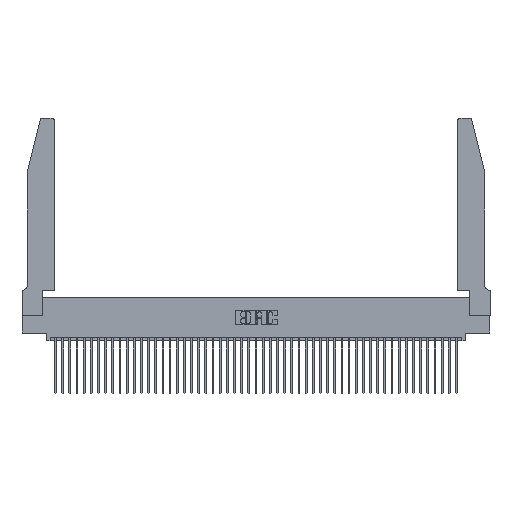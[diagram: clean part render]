
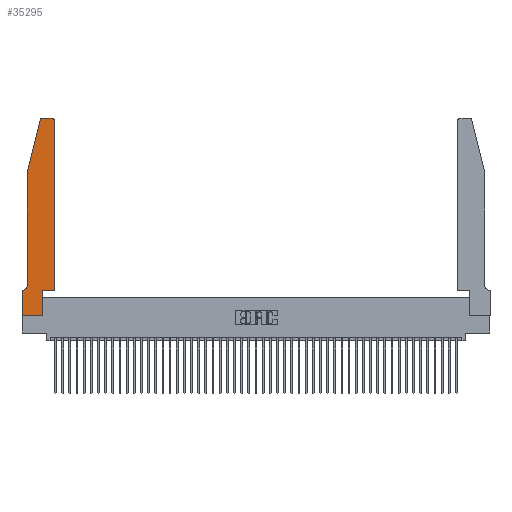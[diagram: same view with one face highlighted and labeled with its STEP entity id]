
A CAD part, top view. The second image highlights one B-rep face of the part: STEP entity #35295.
In plain terms, the highlighted planar face has unit normal (0, 0, 1).
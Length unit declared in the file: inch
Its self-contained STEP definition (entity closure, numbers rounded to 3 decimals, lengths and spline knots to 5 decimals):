
#497 = DIRECTION ( 'NONE',  ( -1., 0., 0. ) ) ;
#1406 = ORIENTED_EDGE ( 'NONE', *, *, #20816, .T. ) ;
#1784 = VECTOR ( 'NONE', #19630, 39.37008 ) ;
#1787 = VECTOR ( 'NONE', #44971, 39.37008 ) ;
#1931 = DIRECTION ( 'NONE',  ( -1., 0., 0. ) ) ;
#2581 = ORIENTED_EDGE ( 'NONE', *, *, #4898, .T. ) ;
#2944 = VERTEX_POINT ( 'NONE', #45969 ) ;
#3312 = CARTESIAN_POINT ( 'NONE',  ( 0., 0., 0.37 ) ) ;
#4297 = ORIENTED_EDGE ( 'NONE', *, *, #11537, .T. ) ;
#4477 = CARTESIAN_POINT ( 'NONE',  ( 0.2605, 2.75, 0.37 ) ) ;
#4898 = EDGE_CURVE ( 'NONE', #16310, #2944, #10769, .T. ) ;
#5303 = VECTOR ( 'NONE', #32879, 39.37008 ) ;
#5355 = CARTESIAN_POINT ( 'NONE',  ( 0.4505, 0.35, 0.37 ) ) ;
#5416 = VERTEX_POINT ( 'NONE', #45116 ) ;
#5475 = ORIENTED_EDGE ( 'NONE', *, *, #32530, .T. ) ;
#5559 = AXIS2_PLACEMENT_3D ( 'NONE', #45998, #24173, #1931 ) ;
#6091 = ORIENTED_EDGE ( 'NONE', *, *, #26059, .T. ) ;
#6346 = CARTESIAN_POINT ( 'NONE',  ( 0.284, 2.72, 0.37 ) ) ;
#6486 = VECTOR ( 'NONE', #18868, 39.37008 ) ;
#7063 = EDGE_LOOP ( 'NONE', ( #30308, #11888, #4297, #5475, #17757, #37172, #1406, #21222, #2581, #34363, #6091, #28052 ) ) ;
#7684 = VERTEX_POINT ( 'NONE', #38017 ) ;
#7776 = CIRCLE ( 'NONE', #23488, 0.03 ) ;
#8033 = EDGE_CURVE ( 'NONE', #5416, #16310, #46451, .T. ) ;
#9741 = LINE ( 'NONE', #5355, #36792 ) ;
#10107 = DIRECTION ( 'NONE',  ( 1., 0., 0. ) ) ;
#10769 = LINE ( 'NONE', #24474, #38880 ) ;
#10992 = CARTESIAN_POINT ( 'NONE',  ( 0.4505, 2.72, 0.37 ) ) ;
#11537 = EDGE_CURVE ( 'NONE', #7684, #43805, #45530, .T. ) ;
#11857 = VECTOR ( 'NONE', #497, 39.37008 ) ;
#11888 = ORIENTED_EDGE ( 'NONE', *, *, #41036, .T. ) ;
#12691 = VECTOR ( 'NONE', #44970, 39.37008 ) ;
#13039 = LINE ( 'NONE', #33638, #11857 ) ;
#13685 = CARTESIAN_POINT ( 'NONE',  ( 0., 0.35, 0.37 ) ) ;
#14522 = CARTESIAN_POINT ( 'NONE',  ( 0.0755, 0.42, 0.37 ) ) ;
#15375 = VERTEX_POINT ( 'NONE', #14522 ) ;
#15816 = CARTESIAN_POINT ( 'NONE',  ( 0.0055, 0.35, 0.37 ) ) ;
#15893 = CARTESIAN_POINT ( 'NONE',  ( 0.0755, 2., 0.37 ) ) ;
#16060 = CARTESIAN_POINT ( 'NONE',  ( 0.284, 2.75, 0.37 ) ) ;
#16310 = VERTEX_POINT ( 'NONE', #17488 ) ;
#16638 = EDGE_CURVE ( 'NONE', #19144, #25656, #13039, .T. ) ;
#17291 = CARTESIAN_POINT ( 'NONE',  ( 0., 0.35, 0.37 ) ) ;
#17488 = CARTESIAN_POINT ( 'NONE',  ( 0.2865, 0., 0.37 ) ) ;
#17757 = ORIENTED_EDGE ( 'NONE', *, *, #29373, .T. ) ;
#18868 = DIRECTION ( 'NONE',  ( -0.239, -0.971, 0. ) ) ;
#19128 = CIRCLE ( 'NONE', #46783, 0.03 ) ;
#19144 = VERTEX_POINT ( 'NONE', #15816 ) ;
#19630 = DIRECTION ( 'NONE',  ( 0., -1., 0. ) ) ;
#20816 = EDGE_CURVE ( 'NONE', #25656, #5416, #23893, .T. ) ;
#20916 = DIRECTION ( 'NONE',  ( 0., 0., 1. ) ) ;
#21017 = DIRECTION ( 'NONE',  ( 0., 0., 1. ) ) ;
#21222 = ORIENTED_EDGE ( 'NONE', *, *, #8033, .T. ) ;
#21611 = LINE ( 'NONE', #15893, #1784 ) ;
#22390 = VERTEX_POINT ( 'NONE', #16060 ) ;
#23488 = AXIS2_PLACEMENT_3D ( 'NONE', #42720, #20916, #46395 ) ;
#23893 = LINE ( 'NONE', #3312, #5303 ) ;
#24173 = DIRECTION ( 'NONE',  ( 0., 0., -1. ) ) ;
#24474 = CARTESIAN_POINT ( 'NONE',  ( 0.2865, 0.35, 0.37 ) ) ;
#25421 = DIRECTION ( 'NONE',  ( 1., 0., 0. ) ) ;
#25656 = VERTEX_POINT ( 'NONE', #13685 ) ;
#26059 = EDGE_CURVE ( 'NONE', #31080, #30648, #31266, .T. ) ;
#27065 = VECTOR ( 'NONE', #25421, 39.37008 ) ;
#28052 = ORIENTED_EDGE ( 'NONE', *, *, #36757, .T. ) ;
#28691 = VERTEX_POINT ( 'NONE', #37899 ) ;
#29373 = EDGE_CURVE ( 'NONE', #15375, #19144, #43479, .T. ) ;
#29726 = CARTESIAN_POINT ( 'NONE',  ( 0.0755, 2., 0.37 ) ) ;
#30308 = ORIENTED_EDGE ( 'NONE', *, *, #34353, .T. ) ;
#30330 = CARTESIAN_POINT ( 'NONE',  ( 0.4505, 0.35, 0.37 ) ) ;
#30648 = VERTEX_POINT ( 'NONE', #10992 ) ;
#31073 = LINE ( 'NONE', #4477, #12691 ) ;
#31080 = VERTEX_POINT ( 'NONE', #43634 ) ;
#31266 = LINE ( 'NONE', #30330, #1787 ) ;
#32134 = DIRECTION ( 'NONE',  ( 0., 0., 1. ) ) ;
#32530 = EDGE_CURVE ( 'NONE', #43805, #15375, #21611, .T. ) ;
#32879 = DIRECTION ( 'NONE',  ( 0., -1., 0. ) ) ;
#33638 = CARTESIAN_POINT ( 'NONE',  ( 0.0755, 0.35, 0.37 ) ) ;
#34353 = EDGE_CURVE ( 'NONE', #28691, #22390, #31073, .T. ) ;
#34363 = ORIENTED_EDGE ( 'NONE', *, *, #46418, .T. ) ;
#34859 = DIRECTION ( 'NONE',  ( 1., 0., 0. ) ) ;
#35295 = ADVANCED_FACE ( 'NONE', ( #40685 ), #39178, .T. ) ;
#36757 = EDGE_CURVE ( 'NONE', #30648, #28691, #7776, .T. ) ;
#36792 = VECTOR ( 'NONE', #34859, 39.37008 ) ;
#36900 = CARTESIAN_POINT ( 'NONE',  ( 0., 0., 0.37 ) ) ;
#36986 = CARTESIAN_POINT ( 'NONE',  ( 0.0755, 2., 0.37 ) ) ;
#37172 = ORIENTED_EDGE ( 'NONE', *, *, #16638, .T. ) ;
#37899 = CARTESIAN_POINT ( 'NONE',  ( 0.4205, 2.75, 0.37 ) ) ;
#38017 = CARTESIAN_POINT ( 'NONE',  ( 0.25487, 2.72718, 0.37 ) ) ;
#38880 = VECTOR ( 'NONE', #38965, 39.37008 ) ;
#38965 = DIRECTION ( 'NONE',  ( 0., 1., 0. ) ) ;
#39178 = PLANE ( 'NONE',  #45086 ) ;
#40685 = FACE_OUTER_BOUND ( 'NONE', #7063, .T. ) ;
#41036 = EDGE_CURVE ( 'NONE', #22390, #7684, #19128, .T. ) ;
#42720 = CARTESIAN_POINT ( 'NONE',  ( 0.4205, 2.72, 0.37 ) ) ;
#43479 = CIRCLE ( 'NONE', #5559, 0.07 ) ;
#43634 = CARTESIAN_POINT ( 'NONE',  ( 0.4505, 0.35, 0.37 ) ) ;
#43805 = VERTEX_POINT ( 'NONE', #36986 ) ;
#44970 = DIRECTION ( 'NONE',  ( -1., 0., 0. ) ) ;
#44971 = DIRECTION ( 'NONE',  ( 0., 1., 0. ) ) ;
#45086 = AXIS2_PLACEMENT_3D ( 'NONE', #17291, #21017, #46497 ) ;
#45116 = CARTESIAN_POINT ( 'NONE',  ( 0., 0., 0.37 ) ) ;
#45530 = LINE ( 'NONE', #29726, #6486 ) ;
#45969 = CARTESIAN_POINT ( 'NONE',  ( 0.2865, 0.35, 0.37 ) ) ;
#45998 = CARTESIAN_POINT ( 'NONE',  ( 0.0055, 0.42, 0.37 ) ) ;
#46395 = DIRECTION ( 'NONE',  ( 1., 0., 0. ) ) ;
#46418 = EDGE_CURVE ( 'NONE', #2944, #31080, #9741, .T. ) ;
#46451 = LINE ( 'NONE', #36900, #27065 ) ;
#46497 = DIRECTION ( 'NONE',  ( 1., 0., 0. ) ) ;
#46783 = AXIS2_PLACEMENT_3D ( 'NONE', #6346, #32134, #10107 ) ;
